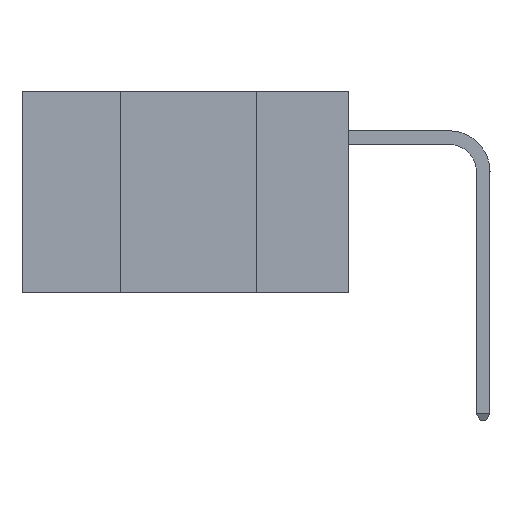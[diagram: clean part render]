
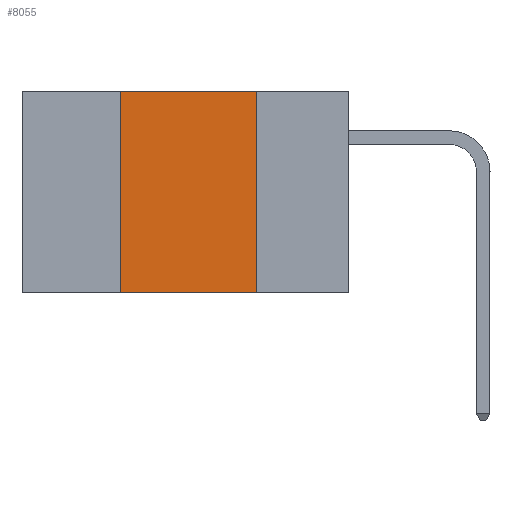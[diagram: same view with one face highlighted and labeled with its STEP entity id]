
A CAD part, left-side view. The second image highlights one B-rep face of the part: STEP entity #8055.
In plain terms, the highlighted planar face has unit normal (-1, 0, 0).
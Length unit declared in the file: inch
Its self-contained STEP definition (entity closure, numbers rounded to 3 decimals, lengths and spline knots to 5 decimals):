
#26 = CARTESIAN_POINT ( 'NONE',  ( 0., 0.17, 0. ) ) ;
#40 = CARTESIAN_POINT ( 'NONE',  ( 0., 0.42, 0. ) ) ;
#168 = LINE ( 'NONE', #26, #6574 ) ;
#469 = DIRECTION ( 'NONE',  ( 1., 0., 0. ) ) ;
#684 = CARTESIAN_POINT ( 'NONE',  ( 0., 0.42, -0.37 ) ) ;
#1640 = CARTESIAN_POINT ( 'NONE',  ( 0., 0.6, -0.37 ) ) ;
#1937 = EDGE_CURVE ( 'NONE', #8927, #8633, #9661, .T. ) ;
#2705 = DIRECTION ( 'NONE',  ( 0., 0., -1. ) ) ;
#2830 = EDGE_LOOP ( 'NONE', ( #3891, #5076, #5278, #13367 ) ) ;
#2831 = AXIS2_PLACEMENT_3D ( 'NONE', #5573, #469, #9290 ) ;
#3651 = DIRECTION ( 'NONE',  ( 0., -1., 0. ) ) ;
#3891 = ORIENTED_EDGE ( 'NONE', *, *, #12768, .F. ) ;
#4173 = VERTEX_POINT ( 'NONE', #14829 ) ;
#4407 = LINE ( 'NONE', #1640, #13634 ) ;
#5076 = ORIENTED_EDGE ( 'NONE', *, *, #6656, .F. ) ;
#5278 = ORIENTED_EDGE ( 'NONE', *, *, #1937, .F. ) ;
#5573 = CARTESIAN_POINT ( 'NONE',  ( 0., 0.6, 0. ) ) ;
#6574 = VECTOR ( 'NONE', #2705, 39.37008 ) ;
#6656 = EDGE_CURVE ( 'NONE', #8633, #4173, #9592, .T. ) ;
#8055 = ADVANCED_FACE ( 'NONE', ( #13062 ), #8089, .F. ) ;
#8089 = PLANE ( 'NONE',  #2831 ) ;
#8633 = VERTEX_POINT ( 'NONE', #40 ) ;
#8927 = VERTEX_POINT ( 'NONE', #684 ) ;
#9290 = DIRECTION ( 'NONE',  ( 0., 0., -1. ) ) ;
#9592 = LINE ( 'NONE', #9805, #12385 ) ;
#9661 = LINE ( 'NONE', #12072, #15434 ) ;
#9805 = CARTESIAN_POINT ( 'NONE',  ( 0., 0.6, 0. ) ) ;
#11900 = VERTEX_POINT ( 'NONE', #14486 ) ;
#12015 = DIRECTION ( 'NONE',  ( 0., 0., 1. ) ) ;
#12072 = CARTESIAN_POINT ( 'NONE',  ( 0., 0.42, 0. ) ) ;
#12385 = VECTOR ( 'NONE', #3651, 39.37008 ) ;
#12737 = DIRECTION ( 'NONE',  ( 0., -1., 0. ) ) ;
#12768 = EDGE_CURVE ( 'NONE', #4173, #11900, #168, .T. ) ;
#13062 = FACE_OUTER_BOUND ( 'NONE', #2830, .T. ) ;
#13367 = ORIENTED_EDGE ( 'NONE', *, *, #14795, .T. ) ;
#13634 = VECTOR ( 'NONE', #12737, 39.37008 ) ;
#14486 = CARTESIAN_POINT ( 'NONE',  ( 0., 0.17, -0.37 ) ) ;
#14795 = EDGE_CURVE ( 'NONE', #8927, #11900, #4407, .T. ) ;
#14829 = CARTESIAN_POINT ( 'NONE',  ( 0., 0.17, 0. ) ) ;
#15434 = VECTOR ( 'NONE', #12015, 39.37008 ) ;
